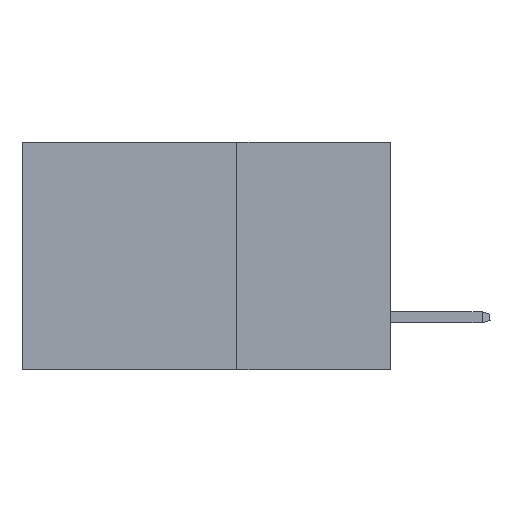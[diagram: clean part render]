
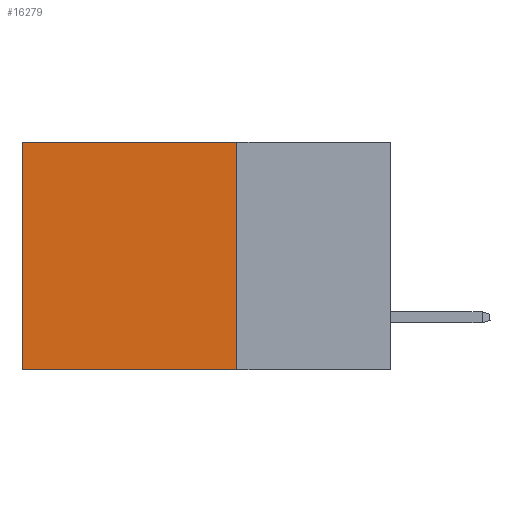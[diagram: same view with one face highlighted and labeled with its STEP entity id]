
A CAD part, left-side view. The second image highlights one B-rep face of the part: STEP entity #16279.
In plain terms, the highlighted planar face has unit normal (-1, 0, 0).
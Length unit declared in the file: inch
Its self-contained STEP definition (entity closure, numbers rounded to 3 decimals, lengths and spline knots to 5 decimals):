
#509 = CARTESIAN_POINT ( 'NONE',  ( 0.2875, 0.25, 0. ) ) ;
#1180 = CARTESIAN_POINT ( 'NONE',  ( 0.2875, 0.25, -0.37 ) ) ;
#1510 = ORIENTED_EDGE ( 'NONE', *, *, #12047, .F. ) ;
#5278 = LINE ( 'NONE', #509, #22094 ) ;
#9685 = VERTEX_POINT ( 'NONE', #15210 ) ;
#10070 = EDGE_CURVE ( 'NONE', #19124, #24474, #15424, .T. ) ;
#10553 = DIRECTION ( 'NONE',  ( 1., 0., 0. ) ) ;
#11374 = LINE ( 'NONE', #36576, #12332 ) ;
#11477 = EDGE_CURVE ( 'NONE', #24474, #32153, #11374, .T. ) ;
#12047 = EDGE_CURVE ( 'NONE', #19124, #9685, #5278, .T. ) ;
#12332 = VECTOR ( 'NONE', #14669, 39.37008 ) ;
#12352 = FACE_OUTER_BOUND ( 'NONE', #17238, .T. ) ;
#13427 = VECTOR ( 'NONE', #29324, 39.37008 ) ;
#14669 = DIRECTION ( 'NONE',  ( 0., 0., -1. ) ) ;
#15210 = CARTESIAN_POINT ( 'NONE',  ( 0.2875, 0.25, -0.37 ) ) ;
#15424 = LINE ( 'NONE', #19975, #13427 ) ;
#16279 = ADVANCED_FACE ( 'NONE', ( #12352 ), #29349, .F. ) ;
#16721 = CARTESIAN_POINT ( 'NONE',  ( 0.2875, 0.25, 0. ) ) ;
#17238 = EDGE_LOOP ( 'NONE', ( #22478, #32400, #1510, #31735 ) ) ;
#19124 = VERTEX_POINT ( 'NONE', #29991 ) ;
#19826 = VECTOR ( 'NONE', #20208, 39.37008 ) ;
#19975 = CARTESIAN_POINT ( 'NONE',  ( 0.2875, 0.25, 0. ) ) ;
#20208 = DIRECTION ( 'NONE',  ( 0., 1., 0. ) ) ;
#22094 = VECTOR ( 'NONE', #38301, 39.37008 ) ;
#22478 = ORIENTED_EDGE ( 'NONE', *, *, #11477, .T. ) ;
#24474 = VERTEX_POINT ( 'NONE', #34264 ) ;
#28173 = LINE ( 'NONE', #1180, #19826 ) ;
#29192 = CARTESIAN_POINT ( 'NONE',  ( 0.2875, 0.6, -0.37 ) ) ;
#29324 = DIRECTION ( 'NONE',  ( 0., 1., 0. ) ) ;
#29349 = PLANE ( 'NONE',  #40055 ) ;
#29991 = CARTESIAN_POINT ( 'NONE',  ( 0.2875, 0.25, 0. ) ) ;
#31735 = ORIENTED_EDGE ( 'NONE', *, *, #10070, .T. ) ;
#32153 = VERTEX_POINT ( 'NONE', #29192 ) ;
#32400 = ORIENTED_EDGE ( 'NONE', *, *, #37717, .F. ) ;
#32474 = DIRECTION ( 'NONE',  ( 0., 0., -1. ) ) ;
#34264 = CARTESIAN_POINT ( 'NONE',  ( 0.2875, 0.6, 0. ) ) ;
#36576 = CARTESIAN_POINT ( 'NONE',  ( 0.2875, 0.6, 0. ) ) ;
#37717 = EDGE_CURVE ( 'NONE', #9685, #32153, #28173, .T. ) ;
#38301 = DIRECTION ( 'NONE',  ( 0., 0., -1. ) ) ;
#40055 = AXIS2_PLACEMENT_3D ( 'NONE', #16721, #10553, #32474 ) ;
